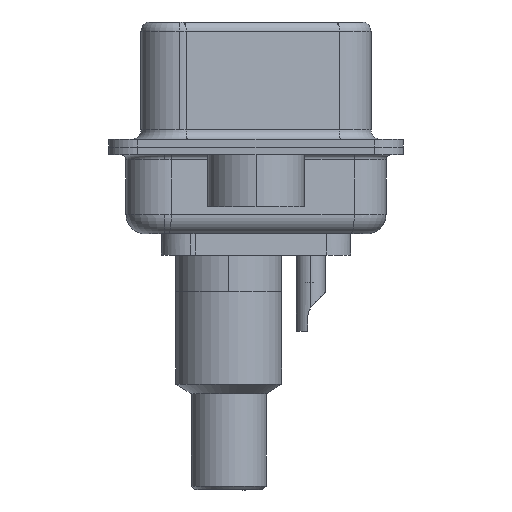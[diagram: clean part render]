
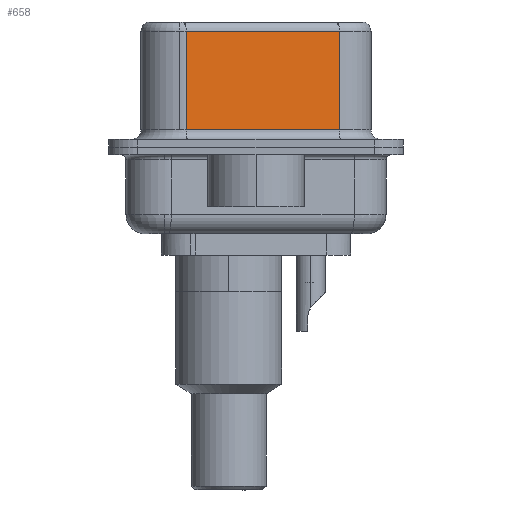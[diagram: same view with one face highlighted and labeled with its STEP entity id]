
A CAD part, left-side view. The second image highlights one B-rep face of the part: STEP entity #658.
In plain terms, the highlighted planar face has unit normal (-0.985, -0.174, 0).
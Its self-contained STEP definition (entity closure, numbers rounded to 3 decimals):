
#658 = ADVANCED_FACE ( 'NONE', ( #8996 ), #19385, .F. ) ;
#1214 = ORIENTED_EDGE ( 'NONE', *, *, #5096, .T. ) ;
#2453 = LINE ( 'NONE', #6741, #21987 ) ;
#2627 = CARTESIAN_POINT ( 'NONE',  ( 5.132, -4.322, 6.52 ) ) ;
#3029 = EDGE_CURVE ( 'NONE', #10502, #9407, #10028, .T. ) ;
#4782 = VERTEX_POINT ( 'NONE', #23633 ) ;
#5096 = EDGE_CURVE ( 'NONE', #4782, #10502, #9943, .T. ) ;
#5591 = VECTOR ( 'NONE', #17008, 1000. ) ;
#6522 = AXIS2_PLACEMENT_3D ( 'NONE', #2627, #14663, #14801 ) ;
#6741 = CARTESIAN_POINT ( 'NONE',  ( 5.132, -4.322, 6.52 ) ) ;
#6825 = EDGE_CURVE ( 'NONE', #11414, #9407, #2453, .T. ) ;
#7247 = LINE ( 'NONE', #16992, #11629 ) ;
#8996 = FACE_OUTER_BOUND ( 'NONE', #19117, .T. ) ;
#9198 = CARTESIAN_POINT ( 'NONE',  ( 5.132, -4.322, 0.9 ) ) ;
#9407 = VERTEX_POINT ( 'NONE', #9198 ) ;
#9836 = CARTESIAN_POINT ( 'NONE',  ( 3.73, 3.628, 6.52 ) ) ;
#9943 = LINE ( 'NONE', #9836, #18201 ) ;
#10028 = LINE ( 'NONE', #22967, #5591 ) ;
#10502 = VERTEX_POINT ( 'NONE', #23420 ) ;
#11414 = VERTEX_POINT ( 'NONE', #22311 ) ;
#11629 = VECTOR ( 'NONE', #22747, 1000. ) ;
#12556 = DIRECTION ( 'NONE',  ( 0., 0., -1. ) ) ;
#14224 = ORIENTED_EDGE ( 'NONE', *, *, #3029, .T. ) ;
#14663 = DIRECTION ( 'NONE',  ( 0.985, 0.174, 0. ) ) ;
#14801 = DIRECTION ( 'NONE',  ( -0.174, 0.985, 0. ) ) ;
#16868 = ORIENTED_EDGE ( 'NONE', *, *, #6825, .F. ) ;
#16992 = CARTESIAN_POINT ( 'NONE',  ( 5.132, -4.322, 6.02 ) ) ;
#17008 = DIRECTION ( 'NONE',  ( 0.174, -0.985, 0. ) ) ;
#17552 = EDGE_CURVE ( 'NONE', #11414, #4782, #7247, .T. ) ;
#18201 = VECTOR ( 'NONE', #21812, 1000. ) ;
#18407 = ORIENTED_EDGE ( 'NONE', *, *, #17552, .T. ) ;
#19117 = EDGE_LOOP ( 'NONE', ( #16868, #18407, #1214, #14224 ) ) ;
#19385 = PLANE ( 'NONE',  #6522 ) ;
#21812 = DIRECTION ( 'NONE',  ( 0., 0., -1. ) ) ;
#21987 = VECTOR ( 'NONE', #12556, 1000. ) ;
#22311 = CARTESIAN_POINT ( 'NONE',  ( 5.132, -4.322, 6.02 ) ) ;
#22747 = DIRECTION ( 'NONE',  ( -0.174, 0.985, 0. ) ) ;
#22967 = CARTESIAN_POINT ( 'NONE',  ( 5.132, -4.322, 0.9 ) ) ;
#23420 = CARTESIAN_POINT ( 'NONE',  ( 3.73, 3.628, 0.9 ) ) ;
#23633 = CARTESIAN_POINT ( 'NONE',  ( 3.73, 3.628, 6.02 ) ) ;
